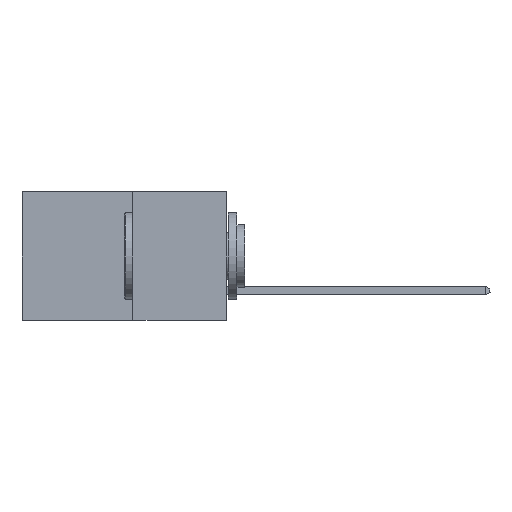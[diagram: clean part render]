
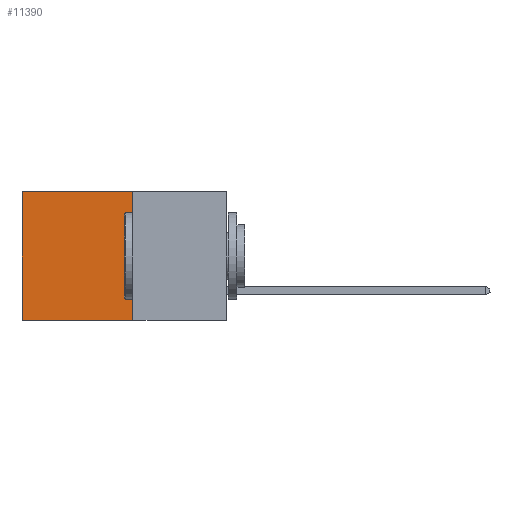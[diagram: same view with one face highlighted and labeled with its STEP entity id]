
A CAD part, left-side view. The second image highlights one B-rep face of the part: STEP entity #11390.
In plain terms, the highlighted planar face has unit normal (-1, 0, 0).
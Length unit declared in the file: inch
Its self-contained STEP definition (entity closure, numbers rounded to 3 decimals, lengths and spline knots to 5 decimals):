
#120 = VERTEX_POINT ( 'NONE', #14567 ) ;
#1346 = LINE ( 'NONE', #16132, #24269 ) ;
#1599 = CARTESIAN_POINT ( 'NONE',  ( 0.277, 0.59, -0.37 ) ) ;
#1876 = ORIENTED_EDGE ( 'NONE', *, *, #26534, .F. ) ;
#2149 = DIRECTION ( 'NONE',  ( 1., 0., 0. ) ) ;
#3321 = ORIENTED_EDGE ( 'NONE', *, *, #17677, .T. ) ;
#3968 = VERTEX_POINT ( 'NONE', #16762 ) ;
#5561 = LINE ( 'NONE', #18847, #16017 ) ;
#5880 = VERTEX_POINT ( 'NONE', #1599 ) ;
#9583 = DIRECTION ( 'NONE',  ( 0., 1., 0. ) ) ;
#9668 = DIRECTION ( 'NONE',  ( 0., 0., -1. ) ) ;
#9899 = VECTOR ( 'NONE', #12601, 39.37008 ) ;
#11390 = ADVANCED_FACE ( 'NONE', ( #25318 ), #22046, .F. ) ;
#11604 = EDGE_CURVE ( 'NONE', #120, #5880, #1346, .T. ) ;
#11726 = ORIENTED_EDGE ( 'NONE', *, *, #11604, .F. ) ;
#12601 = DIRECTION ( 'NONE',  ( 0., 1., 0. ) ) ;
#14170 = VERTEX_POINT ( 'NONE', #25590 ) ;
#14457 = DIRECTION ( 'NONE',  ( 0., 0., -1. ) ) ;
#14567 = CARTESIAN_POINT ( 'NONE',  ( 0.277, 0.27, -0.37 ) ) ;
#15780 = LINE ( 'NONE', #22898, #27336 ) ;
#16017 = VECTOR ( 'NONE', #14457, 39.37008 ) ;
#16132 = CARTESIAN_POINT ( 'NONE',  ( 0.277, 0.27, -0.37 ) ) ;
#16762 = CARTESIAN_POINT ( 'NONE',  ( 0.277, 0.27, 0. ) ) ;
#16977 = CARTESIAN_POINT ( 'NONE',  ( 0.277, 0.27, 0. ) ) ;
#17677 = EDGE_CURVE ( 'NONE', #3968, #14170, #22311, .T. ) ;
#17753 = DIRECTION ( 'NONE',  ( 0., 0., -1. ) ) ;
#18847 = CARTESIAN_POINT ( 'NONE',  ( 0.277, 0.27, -0.37 ) ) ;
#20778 = EDGE_LOOP ( 'NONE', ( #28422, #11726, #1876, #3321 ) ) ;
#22046 = PLANE ( 'NONE',  #22455 ) ;
#22311 = LINE ( 'NONE', #16977, #9899 ) ;
#22455 = AXIS2_PLACEMENT_3D ( 'NONE', #26408, #2149, #17753 ) ;
#22898 = CARTESIAN_POINT ( 'NONE',  ( 0.277, 0.59, -0.37 ) ) ;
#24269 = VECTOR ( 'NONE', #9583, 39.37008 ) ;
#24641 = EDGE_CURVE ( 'NONE', #14170, #5880, #15780, .T. ) ;
#25318 = FACE_OUTER_BOUND ( 'NONE', #20778, .T. ) ;
#25590 = CARTESIAN_POINT ( 'NONE',  ( 0.277, 0.59, 0. ) ) ;
#26408 = CARTESIAN_POINT ( 'NONE',  ( 0.277, 0.27, -0.37 ) ) ;
#26534 = EDGE_CURVE ( 'NONE', #3968, #120, #5561, .T. ) ;
#27336 = VECTOR ( 'NONE', #9668, 39.37008 ) ;
#28422 = ORIENTED_EDGE ( 'NONE', *, *, #24641, .T. ) ;
